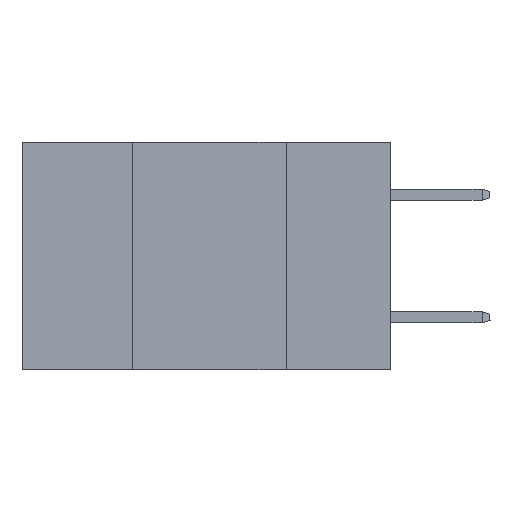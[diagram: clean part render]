
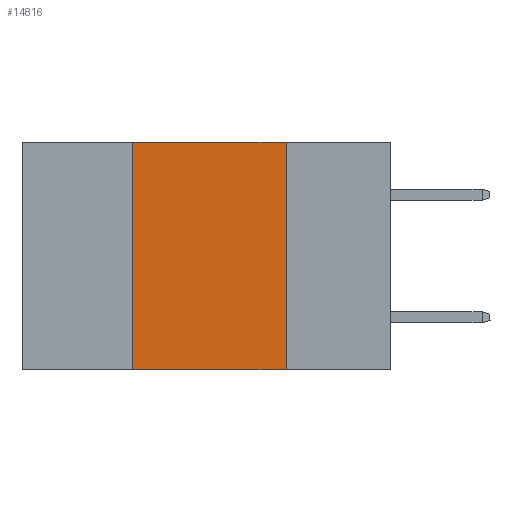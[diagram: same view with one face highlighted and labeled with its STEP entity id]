
A CAD part, left-side view. The second image highlights one B-rep face of the part: STEP entity #14816.
In plain terms, the highlighted planar face has unit normal (-1, 0, 0).
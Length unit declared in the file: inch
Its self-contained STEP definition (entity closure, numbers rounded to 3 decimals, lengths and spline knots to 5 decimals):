
#1827 = EDGE_CURVE ( 'NONE', #13741, #10222, #10749, .T. ) ;
#1964 = VECTOR ( 'NONE', #14213, 39.37008 ) ;
#2312 = CARTESIAN_POINT ( 'NONE',  ( 0., 0.42, 0. ) ) ;
#2446 = EDGE_CURVE ( 'NONE', #10674, #5083, #9845, .T. ) ;
#2810 = ORIENTED_EDGE ( 'NONE', *, *, #11741, .F. ) ;
#3132 = DIRECTION ( 'NONE',  ( 0., -1., 0. ) ) ;
#3479 = CARTESIAN_POINT ( 'NONE',  ( 0., 0.17, 0. ) ) ;
#3949 = CARTESIAN_POINT ( 'NONE',  ( 0., 0.6, -0.37 ) ) ;
#4141 = VECTOR ( 'NONE', #9106, 39.37008 ) ;
#5083 = VERTEX_POINT ( 'NONE', #5861 ) ;
#5861 = CARTESIAN_POINT ( 'NONE',  ( 0., 0.17, 0. ) ) ;
#6237 = VECTOR ( 'NONE', #3132, 39.37008 ) ;
#6778 = PLANE ( 'NONE',  #12252 ) ;
#6887 = CARTESIAN_POINT ( 'NONE',  ( 0., 0.42, 0. ) ) ;
#7003 = CARTESIAN_POINT ( 'NONE',  ( 0., 0.6, 0. ) ) ;
#9106 = DIRECTION ( 'NONE',  ( 0., 0., 1. ) ) ;
#9166 = EDGE_CURVE ( 'NONE', #13741, #10674, #10432, .T. ) ;
#9177 = ORIENTED_EDGE ( 'NONE', *, *, #9166, .F. ) ;
#9845 = LINE ( 'NONE', #7003, #6237 ) ;
#10033 = CARTESIAN_POINT ( 'NONE',  ( 0., 0.42, -0.37 ) ) ;
#10222 = VERTEX_POINT ( 'NONE', #12303 ) ;
#10432 = LINE ( 'NONE', #2312, #4141 ) ;
#10674 = VERTEX_POINT ( 'NONE', #6887 ) ;
#10749 = LINE ( 'NONE', #3949, #16594 ) ;
#11541 = EDGE_LOOP ( 'NONE', ( #2810, #13103, #9177, #13567 ) ) ;
#11741 = EDGE_CURVE ( 'NONE', #5083, #10222, #14468, .T. ) ;
#11826 = FACE_OUTER_BOUND ( 'NONE', #11541, .T. ) ;
#12171 = DIRECTION ( 'NONE',  ( 1., 0., 0. ) ) ;
#12252 = AXIS2_PLACEMENT_3D ( 'NONE', #12263, #12171, #13739 ) ;
#12263 = CARTESIAN_POINT ( 'NONE',  ( 0., 0.6, 0. ) ) ;
#12303 = CARTESIAN_POINT ( 'NONE',  ( 0., 0.17, -0.37 ) ) ;
#13103 = ORIENTED_EDGE ( 'NONE', *, *, #2446, .F. ) ;
#13468 = DIRECTION ( 'NONE',  ( 0., -1., 0. ) ) ;
#13567 = ORIENTED_EDGE ( 'NONE', *, *, #1827, .T. ) ;
#13739 = DIRECTION ( 'NONE',  ( 0., 0., -1. ) ) ;
#13741 = VERTEX_POINT ( 'NONE', #10033 ) ;
#14213 = DIRECTION ( 'NONE',  ( 0., 0., -1. ) ) ;
#14468 = LINE ( 'NONE', #3479, #1964 ) ;
#14816 = ADVANCED_FACE ( 'NONE', ( #11826 ), #6778, .F. ) ;
#16594 = VECTOR ( 'NONE', #13468, 39.37008 ) ;
